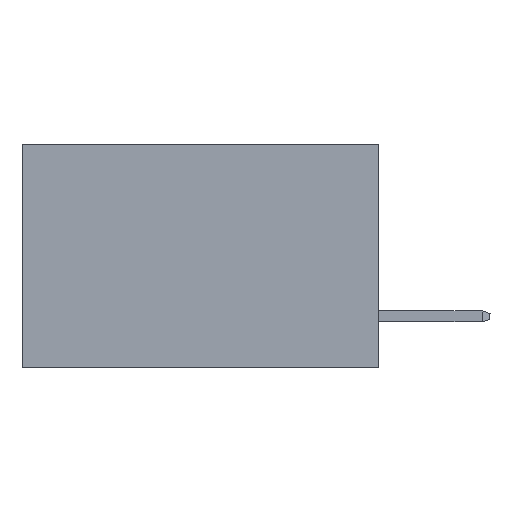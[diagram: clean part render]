
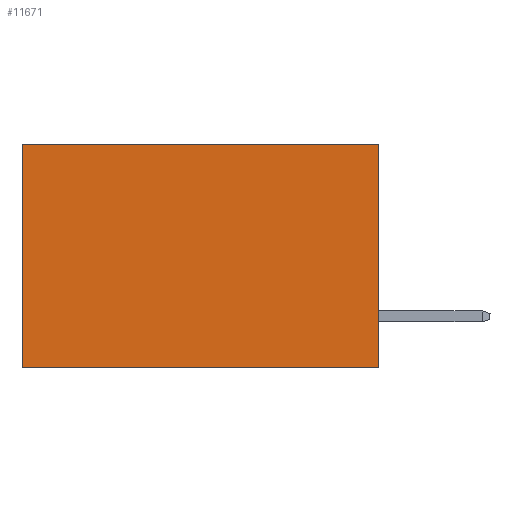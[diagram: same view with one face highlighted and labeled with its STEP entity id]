
A CAD part, left-side view. The second image highlights one B-rep face of the part: STEP entity #11671.
In plain terms, the highlighted planar face has unit normal (-1, 0, 0).
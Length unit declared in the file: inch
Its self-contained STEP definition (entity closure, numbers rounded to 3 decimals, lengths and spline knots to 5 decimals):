
#659 = VERTEX_POINT ( 'NONE', #4096 ) ;
#1002 = DIRECTION ( 'NONE',  ( 0., 0., -1. ) ) ;
#1132 = VECTOR ( 'NONE', #1002, 39.37008 ) ;
#1396 = EDGE_CURVE ( 'NONE', #5745, #10089, #12668, .T. ) ;
#1422 = EDGE_CURVE ( 'NONE', #659, #5745, #1851, .T. ) ;
#1634 = CARTESIAN_POINT ( 'NONE',  ( 0.277, 0., -0.37 ) ) ;
#1851 = LINE ( 'NONE', #12224, #4518 ) ;
#2690 = CARTESIAN_POINT ( 'NONE',  ( 0.277, 0.59, -0.37 ) ) ;
#3286 = CARTESIAN_POINT ( 'NONE',  ( 0.277, 0., -0.37 ) ) ;
#4096 = CARTESIAN_POINT ( 'NONE',  ( 0.277, 0., 0. ) ) ;
#4194 = EDGE_CURVE ( 'NONE', #9340, #10089, #11572, .T. ) ;
#4255 = DIRECTION ( 'NONE',  ( 0., 0., -1. ) ) ;
#4398 = DIRECTION ( 'NONE',  ( 0., 0., -1. ) ) ;
#4518 = VECTOR ( 'NONE', #4255, 39.37008 ) ;
#5240 = DIRECTION ( 'NONE',  ( 0., 1., 0. ) ) ;
#5252 = DIRECTION ( 'NONE',  ( 0., 1., 0. ) ) ;
#5265 = EDGE_LOOP ( 'NONE', ( #11252, #11235, #11086, #11011 ) ) ;
#5745 = VERTEX_POINT ( 'NONE', #1634 ) ;
#6506 = EDGE_CURVE ( 'NONE', #659, #9340, #7771, .T. ) ;
#7771 = LINE ( 'NONE', #8131, #12652 ) ;
#8005 = FACE_OUTER_BOUND ( 'NONE', #5265, .T. ) ;
#8131 = CARTESIAN_POINT ( 'NONE',  ( 0.277, 0., 0. ) ) ;
#9340 = VERTEX_POINT ( 'NONE', #10685 ) ;
#10089 = VERTEX_POINT ( 'NONE', #11824 ) ;
#10173 = DIRECTION ( 'NONE',  ( 1., 0., 0. ) ) ;
#10198 = CARTESIAN_POINT ( 'NONE',  ( 0.277, 0., -0.37 ) ) ;
#10685 = CARTESIAN_POINT ( 'NONE',  ( 0.277, 0.59, 0. ) ) ;
#11011 = ORIENTED_EDGE ( 'NONE', *, *, #6506, .T. ) ;
#11061 = AXIS2_PLACEMENT_3D ( 'NONE', #3286, #10173, #4398 ) ;
#11086 = ORIENTED_EDGE ( 'NONE', *, *, #1422, .F. ) ;
#11235 = ORIENTED_EDGE ( 'NONE', *, *, #1396, .F. ) ;
#11252 = ORIENTED_EDGE ( 'NONE', *, *, #4194, .T. ) ;
#11572 = LINE ( 'NONE', #2690, #1132 ) ;
#11671 = ADVANCED_FACE ( 'NONE', ( #8005 ), #12882, .F. ) ;
#11824 = CARTESIAN_POINT ( 'NONE',  ( 0.277, 0.59, -0.37 ) ) ;
#12224 = CARTESIAN_POINT ( 'NONE',  ( 0.277, 0., -0.37 ) ) ;
#12379 = VECTOR ( 'NONE', #5240, 39.37008 ) ;
#12652 = VECTOR ( 'NONE', #5252, 39.37008 ) ;
#12668 = LINE ( 'NONE', #10198, #12379 ) ;
#12882 = PLANE ( 'NONE',  #11061 ) ;
